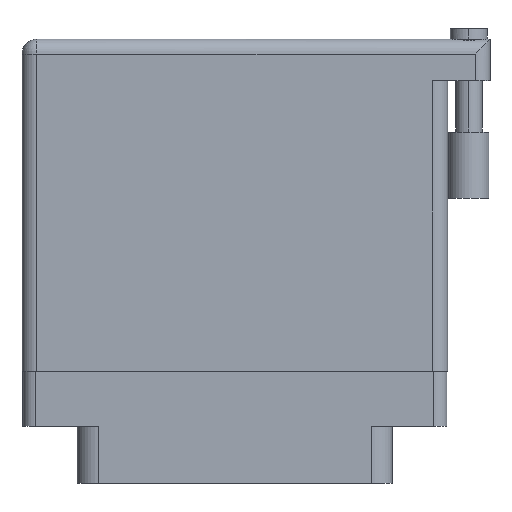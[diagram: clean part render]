
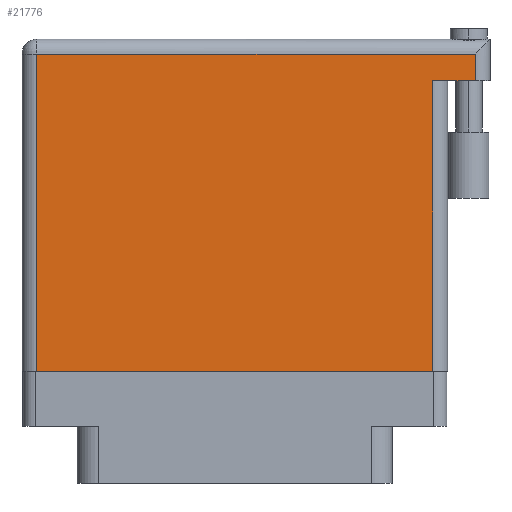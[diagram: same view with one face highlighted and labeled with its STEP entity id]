
A CAD part, front view. The second image highlights one B-rep face of the part: STEP entity #21776.
In plain terms, the highlighted face is planar.
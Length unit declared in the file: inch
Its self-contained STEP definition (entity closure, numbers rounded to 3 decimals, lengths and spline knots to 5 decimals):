
#255 = DIRECTION ( 'NONE',  ( 0., 1., 0. ) ) ;
#410 = VERTEX_POINT ( 'NONE', #3180 ) ;
#1146 = EDGE_CURVE ( 'NONE', #1940, #8951, #23098, .T. ) ;
#1402 = AXIS2_PLACEMENT_3D ( 'NONE', #16700, #5993, #19518 ) ;
#1940 = VERTEX_POINT ( 'NONE', #7021 ) ;
#3074 = LINE ( 'NONE', #18630, #29478 ) ;
#3180 = CARTESIAN_POINT ( 'NONE',  ( 2.138, 1.369, 0. ) ) ;
#3757 = DIRECTION ( 'NONE',  ( 0., 1., 0. ) ) ;
#3930 = ORIENTED_EDGE ( 'NONE', *, *, #17434, .T. ) ;
#4187 = CARTESIAN_POINT ( 'NONE',  ( 1.938, 0., 0. ) ) ;
#4432 = ORIENTED_EDGE ( 'NONE', *, *, #16121, .T. ) ;
#4876 = EDGE_CURVE ( 'NONE', #410, #9013, #3074, .T. ) ;
#5896 = VECTOR ( 'NONE', #255, 39.37008 ) ;
#5993 = DIRECTION ( 'NONE',  ( 0., 0., -1. ) ) ;
#7021 = CARTESIAN_POINT ( 'NONE',  ( 2.138, 1.496, 0. ) ) ;
#7116 = VERTEX_POINT ( 'NONE', #18482 ) ;
#8383 = VECTOR ( 'NONE', #9463, 39.37008 ) ;
#8951 = VERTEX_POINT ( 'NONE', #13124 ) ;
#9013 = VERTEX_POINT ( 'NONE', #13447 ) ;
#9463 = DIRECTION ( 'NONE',  ( 1., 0., 0. ) ) ;
#10107 = LINE ( 'NONE', #33837, #5896 ) ;
#10393 = EDGE_LOOP ( 'NONE', ( #20589, #12745, #29483, #4432, #16449, #3930 ) ) ;
#11161 = DIRECTION ( 'NONE',  ( 0., -1., 0. ) ) ;
#12184 = LINE ( 'NONE', #30880, #8383 ) ;
#12745 = ORIENTED_EDGE ( 'NONE', *, *, #25617, .T. ) ;
#13124 = CARTESIAN_POINT ( 'NONE',  ( 0.07, 1.496, 0. ) ) ;
#13447 = CARTESIAN_POINT ( 'NONE',  ( 1.938, 1.369, 0. ) ) ;
#14400 = DIRECTION ( 'NONE',  ( -1., 0., 0. ) ) ;
#15178 = FACE_OUTER_BOUND ( 'NONE', #10393, .T. ) ;
#16121 = EDGE_CURVE ( 'NONE', #410, #1940, #10107, .T. ) ;
#16449 = ORIENTED_EDGE ( 'NONE', *, *, #1146, .T. ) ;
#16700 = CARTESIAN_POINT ( 'NONE',  ( 0., 1.566, 0. ) ) ;
#17434 = EDGE_CURVE ( 'NONE', #8951, #7116, #24271, .T. ) ;
#18482 = CARTESIAN_POINT ( 'NONE',  ( 0.07, 0., 0. ) ) ;
#18630 = CARTESIAN_POINT ( 'NONE',  ( 2.208, 1.369, 0. ) ) ;
#18686 = LINE ( 'NONE', #29846, #19542 ) ;
#19518 = DIRECTION ( 'NONE',  ( -1., 0., 0. ) ) ;
#19542 = VECTOR ( 'NONE', #3757, 39.37008 ) ;
#20589 = ORIENTED_EDGE ( 'NONE', *, *, #22068, .T. ) ;
#20988 = VECTOR ( 'NONE', #11161, 39.37008 ) ;
#21776 = ADVANCED_FACE ( 'NONE', ( #15178 ), #22308, .F. ) ;
#22068 = EDGE_CURVE ( 'NONE', #7116, #28465, #12184, .T. ) ;
#22308 = PLANE ( 'NONE',  #1402 ) ;
#23098 = LINE ( 'NONE', #32939, #25187 ) ;
#24271 = LINE ( 'NONE', #27211, #20988 ) ;
#25187 = VECTOR ( 'NONE', #14400, 39.37008 ) ;
#25617 = EDGE_CURVE ( 'NONE', #28465, #9013, #18686, .T. ) ;
#27211 = CARTESIAN_POINT ( 'NONE',  ( 0.07, 0., 0. ) ) ;
#28465 = VERTEX_POINT ( 'NONE', #4187 ) ;
#29478 = VECTOR ( 'NONE', #31697, 39.37008 ) ;
#29483 = ORIENTED_EDGE ( 'NONE', *, *, #4876, .F. ) ;
#29846 = CARTESIAN_POINT ( 'NONE',  ( 1.938, 1.369, 0. ) ) ;
#30880 = CARTESIAN_POINT ( 'NONE',  ( 0., 0., 0. ) ) ;
#31697 = DIRECTION ( 'NONE',  ( -1., 0., 0. ) ) ;
#32939 = CARTESIAN_POINT ( 'NONE',  ( 0., 1.496, 0. ) ) ;
#33837 = CARTESIAN_POINT ( 'NONE',  ( 2.138, 1.566, 0. ) ) ;
